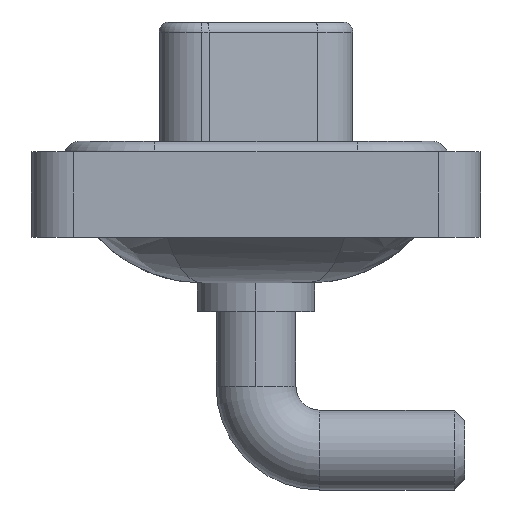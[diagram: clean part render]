
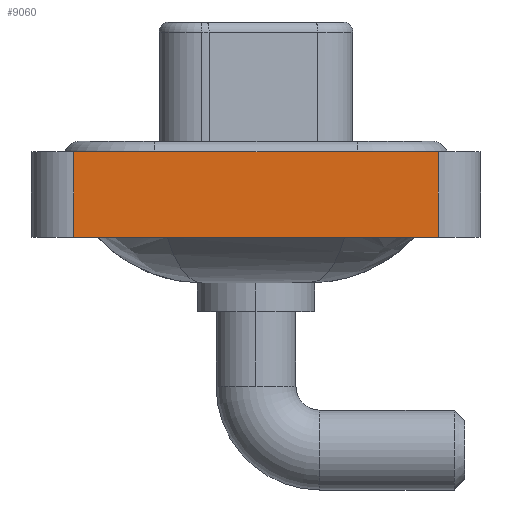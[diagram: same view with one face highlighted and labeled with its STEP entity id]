
A CAD part, left-side view. The second image highlights one B-rep face of the part: STEP entity #9060.
In plain terms, the highlighted planar face has unit normal (-1, 0, 0).
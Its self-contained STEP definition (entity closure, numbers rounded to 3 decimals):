
#90 = EDGE_LOOP ( 'NONE', ( #10363, #7277, #16707, #315 ) ) ;
#315 = ORIENTED_EDGE ( 'NONE', *, *, #7811, .T. ) ;
#1374 = VERTEX_POINT ( 'NONE', #13370 ) ;
#1527 = DIRECTION ( 'NONE',  ( 0., -1., 0. ) ) ;
#2020 = CARTESIAN_POINT ( 'NONE',  ( -7.35, 8.55, 0.4 ) ) ;
#2905 = FACE_OUTER_BOUND ( 'NONE', #90, .T. ) ;
#3889 = CARTESIAN_POINT ( 'NONE',  ( -7.35, -8.55, -3.6 ) ) ;
#4014 = VECTOR ( 'NONE', #17868, 1000. ) ;
#4748 = CARTESIAN_POINT ( 'NONE',  ( -7.35, -8.55, -3.6 ) ) ;
#5351 = LINE ( 'NONE', #6739, #4014 ) ;
#5720 = EDGE_CURVE ( 'NONE', #8303, #1374, #5725, .T. ) ;
#5725 = LINE ( 'NONE', #7205, #10701 ) ;
#6739 = CARTESIAN_POINT ( 'NONE',  ( -7.35, -8.55, 0.4 ) ) ;
#6812 = EDGE_CURVE ( 'NONE', #17909, #1374, #5351, .T. ) ;
#6947 = DIRECTION ( 'NONE',  ( 0., 0., 1. ) ) ;
#7119 = CARTESIAN_POINT ( 'NONE',  ( -7.35, 8.55, -3.6 ) ) ;
#7205 = CARTESIAN_POINT ( 'NONE',  ( -7.35, -8.55, -3.6 ) ) ;
#7277 = ORIENTED_EDGE ( 'NONE', *, *, #6812, .F. ) ;
#7811 = EDGE_CURVE ( 'NONE', #10569, #8303, #14327, .T. ) ;
#8303 = VERTEX_POINT ( 'NONE', #4748 ) ;
#8953 = EDGE_CURVE ( 'NONE', #10569, #17909, #11793, .T. ) ;
#9060 = ADVANCED_FACE ( 'NONE', ( #2905 ), #13717, .T. ) ;
#10363 = ORIENTED_EDGE ( 'NONE', *, *, #5720, .T. ) ;
#10499 = VECTOR ( 'NONE', #1527, 1000. ) ;
#10513 = DIRECTION ( 'NONE',  ( 0., 0., 1. ) ) ;
#10569 = VERTEX_POINT ( 'NONE', #7119 ) ;
#10701 = VECTOR ( 'NONE', #12793, 1000. ) ;
#10883 = AXIS2_PLACEMENT_3D ( 'NONE', #3889, #15057, #6947 ) ;
#11793 = LINE ( 'NONE', #17445, #17282 ) ;
#12793 = DIRECTION ( 'NONE',  ( 0., 0., 1. ) ) ;
#13370 = CARTESIAN_POINT ( 'NONE',  ( -7.35, -8.55, 0.4 ) ) ;
#13717 = PLANE ( 'NONE',  #10883 ) ;
#14327 = LINE ( 'NONE', #15596, #10499 ) ;
#15057 = DIRECTION ( 'NONE',  ( -1., 0., 0. ) ) ;
#15596 = CARTESIAN_POINT ( 'NONE',  ( -7.35, -8.55, -3.6 ) ) ;
#16707 = ORIENTED_EDGE ( 'NONE', *, *, #8953, .F. ) ;
#17282 = VECTOR ( 'NONE', #10513, 1000. ) ;
#17445 = CARTESIAN_POINT ( 'NONE',  ( -7.35, 8.55, -3.6 ) ) ;
#17868 = DIRECTION ( 'NONE',  ( 0., -1., 0. ) ) ;
#17909 = VERTEX_POINT ( 'NONE', #2020 ) ;
